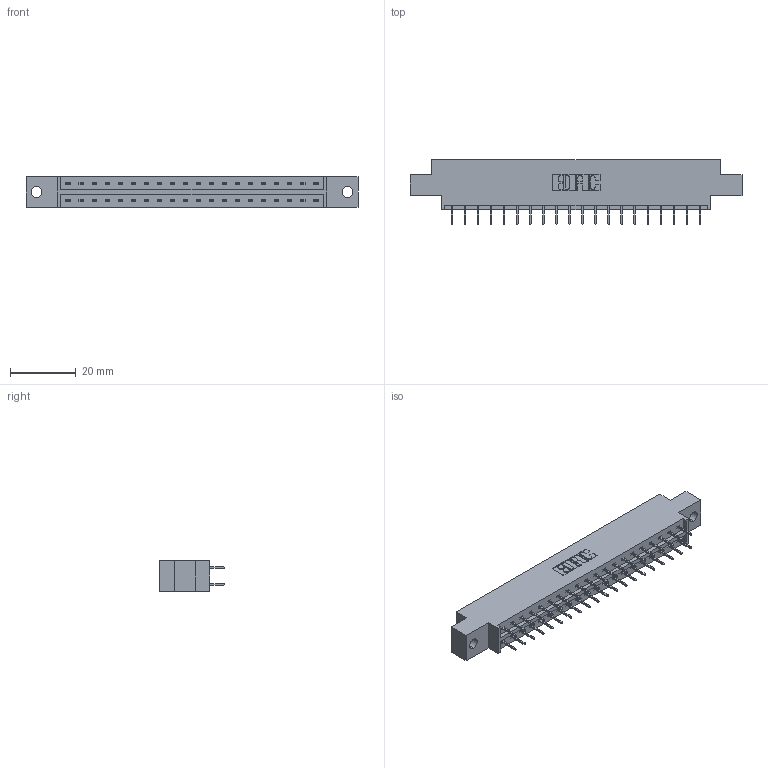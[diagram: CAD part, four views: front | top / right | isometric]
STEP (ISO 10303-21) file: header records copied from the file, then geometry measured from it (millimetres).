
FILE_DESCRIPTION (( 'STEP AP203' ), '1' );
FILE_NAME ('333-040-524-802.STEP', '2018-08-03T13:59:57', ( '' ), ( '' ), 'SwSTEP 2.0', 'SolidWorks 2016', '' );
FILE_SCHEMA (( 'CONFIG_CONTROL_DESIGN' ));
Length unit declared in the file: inch
Products named in the file (3): 333 Part_Offset - .128 Dia; 345-292-001_345-293-124; 333-040-524-802
Assembly tree (41 placements, depth 2):
  333-040-524-802
    333 Part_Offset - .128 Dia
    345-292-001_345-293-124  x40
Bounding box: 100.79 x 19.69 x 9.4 mm (x, y, z)
Volume: 9759 mm3; surface area: 11067 mm2
Topology: 41 solids, 41 shells, 2358 faces, 6683 edges, 4294 vertices
Faces by surface type: plane 1754, cylinder 604
Entity records: 15921 total; most frequent: CARTESIAN_POINT 2666, ORIENTED_EDGE 2602, DIRECTION 2317, EDGE_CURVE 1301, VECTOR 1177, LINE 1177, VERTEX_POINT 862, AXIS2_PLACEMENT_3D 570
